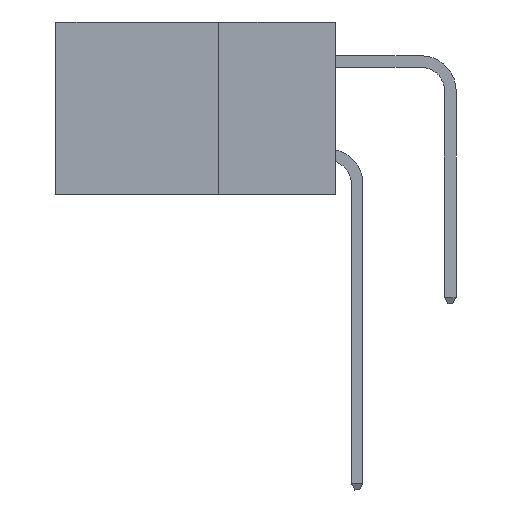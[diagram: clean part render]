
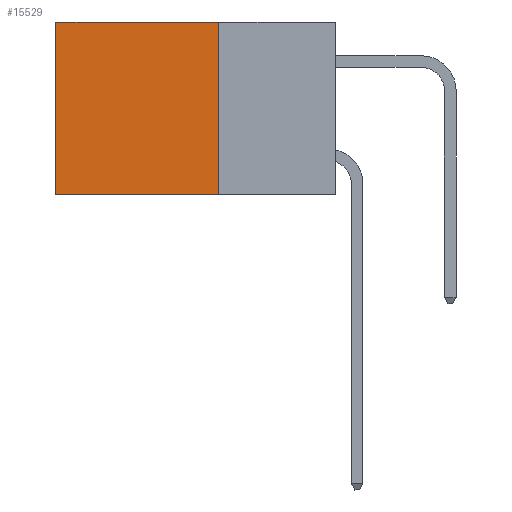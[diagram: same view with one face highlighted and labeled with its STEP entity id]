
A CAD part, left-side view. The second image highlights one B-rep face of the part: STEP entity #15529.
In plain terms, the highlighted planar face has unit normal (-1, 0, 0).
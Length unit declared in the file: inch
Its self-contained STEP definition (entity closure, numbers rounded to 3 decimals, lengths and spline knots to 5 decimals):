
#347 = CARTESIAN_POINT ( 'NONE',  ( 0.2875, 0.25, 0. ) ) ;
#1020 = DIRECTION ( 'NONE',  ( 0., 1., 0. ) ) ;
#2528 = CARTESIAN_POINT ( 'NONE',  ( 0.2875, 0.6, 0. ) ) ;
#2761 = DIRECTION ( 'NONE',  ( 0., 0., -1. ) ) ;
#2821 = FACE_OUTER_BOUND ( 'NONE', #29457, .T. ) ;
#2943 = CARTESIAN_POINT ( 'NONE',  ( 0.2875, 0.25, -0.37 ) ) ;
#3316 = CARTESIAN_POINT ( 'NONE',  ( 0.2875, 0.6, 0. ) ) ;
#3933 = CARTESIAN_POINT ( 'NONE',  ( 0.2875, 0.6, -0.37 ) ) ;
#5952 = ORIENTED_EDGE ( 'NONE', *, *, #33008, .F. ) ;
#6245 = ORIENTED_EDGE ( 'NONE', *, *, #18312, .F. ) ;
#8716 = AXIS2_PLACEMENT_3D ( 'NONE', #347, #11168, #9217 ) ;
#9081 = VERTEX_POINT ( 'NONE', #12097 ) ;
#9217 = DIRECTION ( 'NONE',  ( 0., 0., -1. ) ) ;
#9938 = VECTOR ( 'NONE', #16458, 39.37008 ) ;
#10583 = CARTESIAN_POINT ( 'NONE',  ( 0.2875, 0.25, 0. ) ) ;
#11168 = DIRECTION ( 'NONE',  ( 1., 0., 0. ) ) ;
#11296 = LINE ( 'NONE', #3316, #29051 ) ;
#11481 = DIRECTION ( 'NONE',  ( 0., 0., -1. ) ) ;
#12097 = CARTESIAN_POINT ( 'NONE',  ( 0.2875, 0.25, 0. ) ) ;
#13653 = PLANE ( 'NONE',  #8716 ) ;
#14304 = LINE ( 'NONE', #2943, #9938 ) ;
#14321 = VECTOR ( 'NONE', #2761, 39.37008 ) ;
#14515 = CARTESIAN_POINT ( 'NONE',  ( 0.2875, 0.25, -0.37 ) ) ;
#14984 = VERTEX_POINT ( 'NONE', #2528 ) ;
#15469 = VECTOR ( 'NONE', #1020, 39.37008 ) ;
#15529 = ADVANCED_FACE ( 'NONE', ( #2821 ), #13653, .F. ) ;
#16458 = DIRECTION ( 'NONE',  ( 0., 1., 0. ) ) ;
#16497 = VERTEX_POINT ( 'NONE', #3933 ) ;
#18312 = EDGE_CURVE ( 'NONE', #31481, #16497, #14304, .T. ) ;
#21220 = ORIENTED_EDGE ( 'NONE', *, *, #25114, .T. ) ;
#24641 = CARTESIAN_POINT ( 'NONE',  ( 0.2875, 0.25, 0. ) ) ;
#25072 = EDGE_CURVE ( 'NONE', #14984, #16497, #11296, .T. ) ;
#25114 = EDGE_CURVE ( 'NONE', #9081, #14984, #25342, .T. ) ;
#25342 = LINE ( 'NONE', #24641, #15469 ) ;
#25857 = ORIENTED_EDGE ( 'NONE', *, *, #25072, .T. ) ;
#28780 = LINE ( 'NONE', #10583, #14321 ) ;
#29051 = VECTOR ( 'NONE', #11481, 39.37008 ) ;
#29457 = EDGE_LOOP ( 'NONE', ( #25857, #6245, #5952, #21220 ) ) ;
#31481 = VERTEX_POINT ( 'NONE', #14515 ) ;
#33008 = EDGE_CURVE ( 'NONE', #9081, #31481, #28780, .T. ) ;
